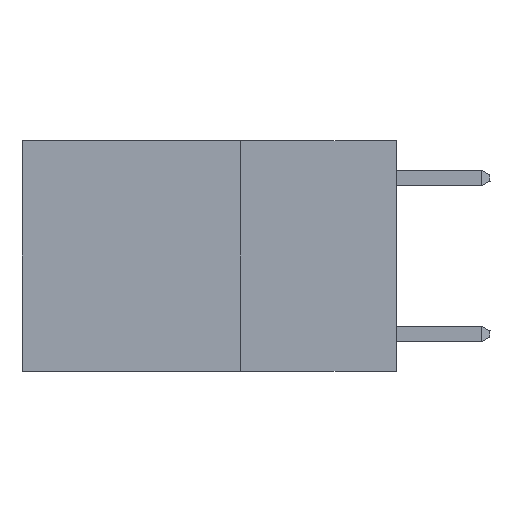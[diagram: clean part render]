
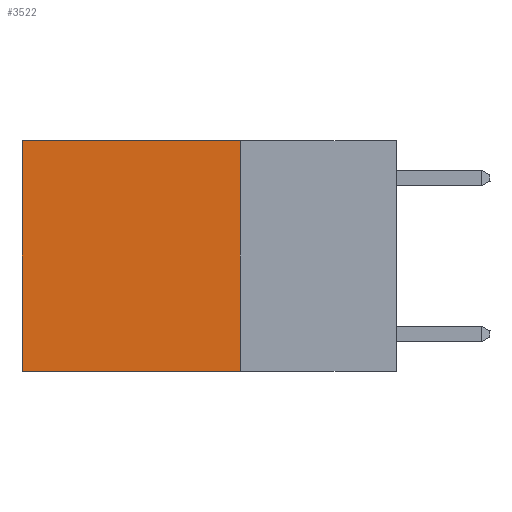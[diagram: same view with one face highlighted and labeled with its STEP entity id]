
A CAD part, left-side view. The second image highlights one B-rep face of the part: STEP entity #3522.
In plain terms, the highlighted planar face has unit normal (-1, 0, 0).
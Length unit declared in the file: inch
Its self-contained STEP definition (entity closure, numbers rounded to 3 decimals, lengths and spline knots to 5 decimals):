
#337 = AXIS2_PLACEMENT_3D ( 'NONE', #2412, #12266, #3335 ) ;
#703 = DIRECTION ( 'NONE',  ( 0., 0., -1. ) ) ;
#726 = ORIENTED_EDGE ( 'NONE', *, *, #9813, .F. ) ;
#1017 = CARTESIAN_POINT ( 'NONE',  ( 0.2625, 0.25, -0.37 ) ) ;
#1964 = EDGE_CURVE ( 'NONE', #2417, #11855, #10380, .T. ) ;
#2412 = CARTESIAN_POINT ( 'NONE',  ( 0.2625, 0.25, 0. ) ) ;
#2417 = VERTEX_POINT ( 'NONE', #12543 ) ;
#2422 = LINE ( 'NONE', #5486, #5210 ) ;
#3335 = DIRECTION ( 'NONE',  ( 0., 0., -1. ) ) ;
#3465 = CARTESIAN_POINT ( 'NONE',  ( 0.2625, 0.6, -0.37 ) ) ;
#3522 = ADVANCED_FACE ( 'NONE', ( #10250 ), #11299, .F. ) ;
#3571 = EDGE_LOOP ( 'NONE', ( #9332, #726, #11782, #5404 ) ) ;
#3650 = CARTESIAN_POINT ( 'NONE',  ( 0.2625, 0.25, 0. ) ) ;
#3770 = VECTOR ( 'NONE', #7482, 39.37008 ) ;
#3825 = CARTESIAN_POINT ( 'NONE',  ( 0.2625, 0.25, -0.37 ) ) ;
#4146 = VERTEX_POINT ( 'NONE', #12807 ) ;
#4711 = EDGE_CURVE ( 'NONE', #2417, #4146, #12098, .T. ) ;
#5000 = VECTOR ( 'NONE', #11781, 39.37008 ) ;
#5210 = VECTOR ( 'NONE', #703, 39.37008 ) ;
#5404 = ORIENTED_EDGE ( 'NONE', *, *, #4711, .T. ) ;
#5486 = CARTESIAN_POINT ( 'NONE',  ( 0.2625, 0.6, 0. ) ) ;
#7233 = VERTEX_POINT ( 'NONE', #3465 ) ;
#7482 = DIRECTION ( 'NONE',  ( 0., 0., -1. ) ) ;
#7844 = LINE ( 'NONE', #3825, #5000 ) ;
#8175 = CARTESIAN_POINT ( 'NONE',  ( 0.2625, 0.25, 0. ) ) ;
#8839 = VECTOR ( 'NONE', #10203, 39.37008 ) ;
#9332 = ORIENTED_EDGE ( 'NONE', *, *, #10197, .T. ) ;
#9813 = EDGE_CURVE ( 'NONE', #11855, #7233, #7844, .T. ) ;
#10197 = EDGE_CURVE ( 'NONE', #4146, #7233, #2422, .T. ) ;
#10203 = DIRECTION ( 'NONE',  ( 0., 1., 0. ) ) ;
#10250 = FACE_OUTER_BOUND ( 'NONE', #3571, .T. ) ;
#10380 = LINE ( 'NONE', #3650, #3770 ) ;
#11299 = PLANE ( 'NONE',  #337 ) ;
#11781 = DIRECTION ( 'NONE',  ( 0., 1., 0. ) ) ;
#11782 = ORIENTED_EDGE ( 'NONE', *, *, #1964, .F. ) ;
#11855 = VERTEX_POINT ( 'NONE', #1017 ) ;
#12098 = LINE ( 'NONE', #8175, #8839 ) ;
#12266 = DIRECTION ( 'NONE',  ( 1., 0., 0. ) ) ;
#12543 = CARTESIAN_POINT ( 'NONE',  ( 0.2625, 0.25, 0. ) ) ;
#12807 = CARTESIAN_POINT ( 'NONE',  ( 0.2625, 0.6, 0. ) ) ;
